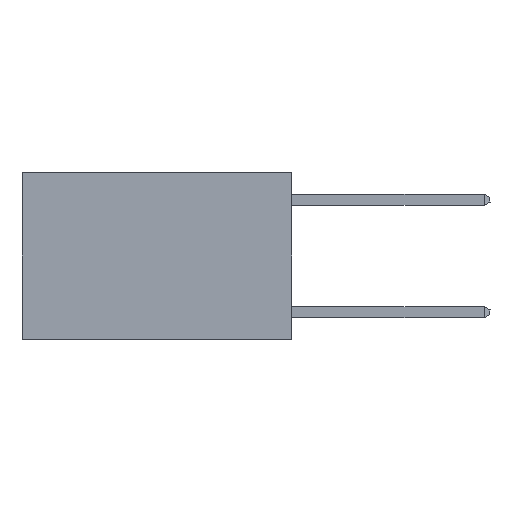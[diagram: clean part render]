
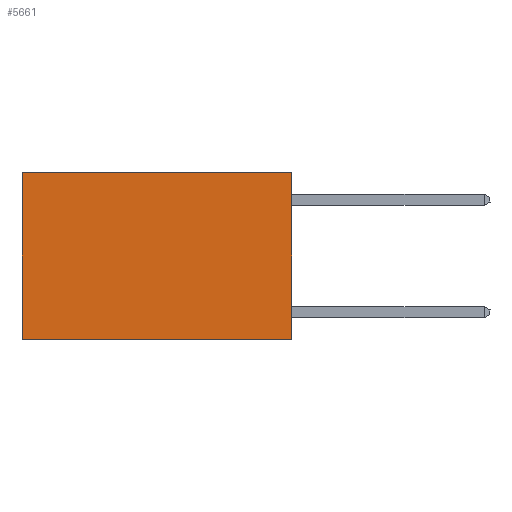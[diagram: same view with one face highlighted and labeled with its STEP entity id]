
A CAD part, left-side view. The second image highlights one B-rep face of the part: STEP entity #5661.
In plain terms, the highlighted planar face has unit normal (-1, 0, 0).
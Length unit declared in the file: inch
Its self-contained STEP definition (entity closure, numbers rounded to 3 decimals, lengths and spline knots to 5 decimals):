
#1285 = ORIENTED_EDGE ( 'NONE', *, *, #9466, .F. ) ;
#1293 = CARTESIAN_POINT ( 'NONE',  ( 0.2625, 0., 0. ) ) ;
#2315 = ORIENTED_EDGE ( 'NONE', *, *, #8412, .F. ) ;
#2647 = CARTESIAN_POINT ( 'NONE',  ( 0.2625, 0., 0. ) ) ;
#3037 = LINE ( 'NONE', #26013, #21378 ) ;
#3689 = LINE ( 'NONE', #8485, #23217 ) ;
#4553 = VERTEX_POINT ( 'NONE', #25676 ) ;
#5527 = AXIS2_PLACEMENT_3D ( 'NONE', #2647, #18460, #8333 ) ;
#5661 = ADVANCED_FACE ( 'NONE', ( #24824 ), #18540, .F. ) ;
#6107 = DIRECTION ( 'NONE',  ( 0., 0., -1. ) ) ;
#6748 = CARTESIAN_POINT ( 'NONE',  ( 0.2625, 0.6, 0. ) ) ;
#8333 = DIRECTION ( 'NONE',  ( 0., 0., -1. ) ) ;
#8412 = EDGE_CURVE ( 'NONE', #19725, #22582, #23606, .T. ) ;
#8485 = CARTESIAN_POINT ( 'NONE',  ( 0.2625, 0., -0.37 ) ) ;
#9171 = ORIENTED_EDGE ( 'NONE', *, *, #14792, .T. ) ;
#9466 = EDGE_CURVE ( 'NONE', #22582, #4553, #3689, .T. ) ;
#9720 = DIRECTION ( 'NONE',  ( 0., 1., 0. ) ) ;
#13951 = CARTESIAN_POINT ( 'NONE',  ( 0.2625, 0., 0. ) ) ;
#14430 = CARTESIAN_POINT ( 'NONE',  ( 0.2625, 0.6, 0. ) ) ;
#14792 = EDGE_CURVE ( 'NONE', #19725, #23270, #3037, .T. ) ;
#16047 = LINE ( 'NONE', #14430, #24711 ) ;
#16784 = VECTOR ( 'NONE', #20190, 39.37008 ) ;
#18460 = DIRECTION ( 'NONE',  ( 1., 0., 0. ) ) ;
#18540 = PLANE ( 'NONE',  #5527 ) ;
#19725 = VERTEX_POINT ( 'NONE', #1293 ) ;
#20190 = DIRECTION ( 'NONE',  ( 0., 0., -1. ) ) ;
#20841 = DIRECTION ( 'NONE',  ( 0., 1., 0. ) ) ;
#21378 = VECTOR ( 'NONE', #9720, 39.37008 ) ;
#22415 = EDGE_LOOP ( 'NONE', ( #24673, #1285, #2315, #9171 ) ) ;
#22502 = CARTESIAN_POINT ( 'NONE',  ( 0.2625, 0., -0.37 ) ) ;
#22582 = VERTEX_POINT ( 'NONE', #22502 ) ;
#23217 = VECTOR ( 'NONE', #20841, 39.37008 ) ;
#23270 = VERTEX_POINT ( 'NONE', #6748 ) ;
#23606 = LINE ( 'NONE', #13951, #16784 ) ;
#24673 = ORIENTED_EDGE ( 'NONE', *, *, #25007, .T. ) ;
#24711 = VECTOR ( 'NONE', #6107, 39.37008 ) ;
#24824 = FACE_OUTER_BOUND ( 'NONE', #22415, .T. ) ;
#25007 = EDGE_CURVE ( 'NONE', #23270, #4553, #16047, .T. ) ;
#25676 = CARTESIAN_POINT ( 'NONE',  ( 0.2625, 0.6, -0.37 ) ) ;
#26013 = CARTESIAN_POINT ( 'NONE',  ( 0.2625, 0., 0. ) ) ;
